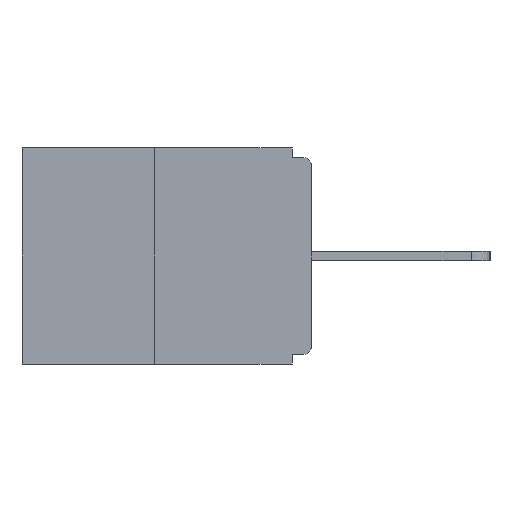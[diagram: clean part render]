
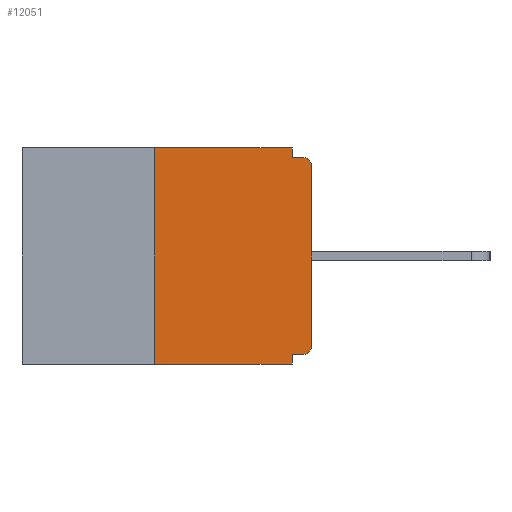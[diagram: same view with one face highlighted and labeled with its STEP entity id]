
A CAD part, left-side view. The second image highlights one B-rep face of the part: STEP entity #12051.
In plain terms, the highlighted planar face has unit normal (-1, 0, 0).
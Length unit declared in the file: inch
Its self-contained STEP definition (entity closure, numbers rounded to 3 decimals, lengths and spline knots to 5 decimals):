
#163 = ORIENTED_EDGE ( 'NONE', *, *, #1763, .F. ) ;
#190 = VERTEX_POINT ( 'NONE', #10523 ) ;
#207 = EDGE_CURVE ( 'NONE', #3106, #6853, #5096, .T. ) ;
#289 = VECTOR ( 'NONE', #5837, 39.37008 ) ;
#712 = DIRECTION ( 'NONE',  ( 0., 0., -1. ) ) ;
#765 = CARTESIAN_POINT ( 'NONE',  ( 0., 0.031, -0.015 ) ) ;
#1212 = EDGE_CURVE ( 'NONE', #190, #12961, #6072, .T. ) ;
#1265 = LINE ( 'NONE', #8754, #4879 ) ;
#1267 = ORIENTED_EDGE ( 'NONE', *, *, #207, .F. ) ;
#1307 = EDGE_CURVE ( 'NONE', #7905, #5545, #8276, .T. ) ;
#1506 = VECTOR ( 'NONE', #12488, 39.37008 ) ;
#1714 = LINE ( 'NONE', #9576, #11235 ) ;
#1763 = EDGE_CURVE ( 'NONE', #7905, #190, #1265, .T. ) ;
#2494 = DIRECTION ( 'NONE',  ( 0., 0., -1. ) ) ;
#2505 = DIRECTION ( 'NONE',  ( 0., 0., -1. ) ) ;
#2756 = CARTESIAN_POINT ( 'NONE',  ( 0., 0., -0.313 ) ) ;
#2762 = LINE ( 'NONE', #11006, #5816 ) ;
#2764 = ORIENTED_EDGE ( 'NONE', *, *, #10537, .F. ) ;
#3025 = ORIENTED_EDGE ( 'NONE', *, *, #3250, .T. ) ;
#3106 = VERTEX_POINT ( 'NONE', #765 ) ;
#3190 = LINE ( 'NONE', #3786, #289 ) ;
#3193 = VECTOR ( 'NONE', #712, 39.37008 ) ;
#3250 = EDGE_CURVE ( 'NONE', #5545, #9030, #11290, .T. ) ;
#3786 = CARTESIAN_POINT ( 'NONE',  ( 0., 0.46, -0.343 ) ) ;
#4188 = CARTESIAN_POINT ( 'NONE',  ( 0., 0.031, 0. ) ) ;
#4225 = DIRECTION ( 'NONE',  ( 0., 0., -1. ) ) ;
#4613 = EDGE_CURVE ( 'NONE', #9030, #6853, #13272, .T. ) ;
#4745 = DIRECTION ( 'NONE',  ( -1., 0., 0. ) ) ;
#4850 = CARTESIAN_POINT ( 'NONE',  ( 0., 0., 0. ) ) ;
#4879 = VECTOR ( 'NONE', #6468, 39.37008 ) ;
#4902 = ORIENTED_EDGE ( 'NONE', *, *, #4613, .T. ) ;
#4992 = CARTESIAN_POINT ( 'NONE',  ( 0., 0., -0.015 ) ) ;
#5096 = LINE ( 'NONE', #4992, #1506 ) ;
#5313 = EDGE_CURVE ( 'NONE', #11545, #3106, #13612, .T. ) ;
#5322 = EDGE_CURVE ( 'NONE', #12980, #11545, #1714, .T. ) ;
#5545 = VERTEX_POINT ( 'NONE', #2756 ) ;
#5580 = DIRECTION ( 'NONE',  ( 0., 0., 1. ) ) ;
#5816 = VECTOR ( 'NONE', #5580, 39.37008 ) ;
#5837 = DIRECTION ( 'NONE',  ( 0., -1., 0. ) ) ;
#5881 = CARTESIAN_POINT ( 'NONE',  ( 0., 0.46, 0. ) ) ;
#5884 = FACE_OUTER_BOUND ( 'NONE', #7782, .T. ) ;
#6072 = LINE ( 'NONE', #9237, #3193 ) ;
#6159 = CARTESIAN_POINT ( 'NONE',  ( 0., 0.031, -0.343 ) ) ;
#6468 = DIRECTION ( 'NONE',  ( 0., 1., 0. ) ) ;
#6846 = CARTESIAN_POINT ( 'NONE',  ( 0., 0.015, -0.03 ) ) ;
#6853 = VERTEX_POINT ( 'NONE', #8956 ) ;
#7450 = DIRECTION ( 'NONE',  ( 0., 0., -1. ) ) ;
#7782 = EDGE_LOOP ( 'NONE', ( #13099, #2764, #8736, #10281, #163, #11491, #3025, #4902, #1267, #11516 ) ) ;
#7905 = VERTEX_POINT ( 'NONE', #12425 ) ;
#8276 = CIRCLE ( 'NONE', #13742, 0.015 ) ;
#8594 = DIRECTION ( 'NONE',  ( 0., -1., 0. ) ) ;
#8736 = ORIENTED_EDGE ( 'NONE', *, *, #10135, .T. ) ;
#8754 = CARTESIAN_POINT ( 'NONE',  ( 0., 0., -0.328 ) ) ;
#8956 = CARTESIAN_POINT ( 'NONE',  ( 0., 0.015, -0.015 ) ) ;
#9006 = PLANE ( 'NONE',  #14054 ) ;
#9030 = VERTEX_POINT ( 'NONE', #11550 ) ;
#9210 = DIRECTION ( 'NONE',  ( 0., 0., 1. ) ) ;
#9237 = CARTESIAN_POINT ( 'NONE',  ( 0., 0.031, -0.343 ) ) ;
#9576 = CARTESIAN_POINT ( 'NONE',  ( 0., 0.46, 0. ) ) ;
#10135 = EDGE_CURVE ( 'NONE', #11312, #12961, #3190, .T. ) ;
#10281 = ORIENTED_EDGE ( 'NONE', *, *, #1212, .F. ) ;
#10442 = VECTOR ( 'NONE', #9210, 39.37008 ) ;
#10523 = CARTESIAN_POINT ( 'NONE',  ( 0., 0.031, -0.328 ) ) ;
#10537 = EDGE_CURVE ( 'NONE', #11312, #12980, #2762, .T. ) ;
#10743 = DIRECTION ( 'NONE',  ( -1., 0., 0. ) ) ;
#11006 = CARTESIAN_POINT ( 'NONE',  ( 0., 0.25, 0. ) ) ;
#11235 = VECTOR ( 'NONE', #8594, 39.37008 ) ;
#11290 = LINE ( 'NONE', #4850, #10442 ) ;
#11312 = VERTEX_POINT ( 'NONE', #12009 ) ;
#11491 = ORIENTED_EDGE ( 'NONE', *, *, #1307, .T. ) ;
#11516 = ORIENTED_EDGE ( 'NONE', *, *, #5313, .F. ) ;
#11545 = VERTEX_POINT ( 'NONE', #12174 ) ;
#11550 = CARTESIAN_POINT ( 'NONE',  ( 0., 0., -0.03 ) ) ;
#11565 = VECTOR ( 'NONE', #7450, 39.37008 ) ;
#11677 = CARTESIAN_POINT ( 'NONE',  ( 0., 0.25, 0. ) ) ;
#11815 = CARTESIAN_POINT ( 'NONE',  ( 0., 0.015, -0.313 ) ) ;
#11878 = AXIS2_PLACEMENT_3D ( 'NONE', #6846, #4745, #2494 ) ;
#12009 = CARTESIAN_POINT ( 'NONE',  ( 0., 0.25, -0.343 ) ) ;
#12051 = ADVANCED_FACE ( 'NONE', ( #5884 ), #9006, .F. ) ;
#12174 = CARTESIAN_POINT ( 'NONE',  ( 0., 0.031, 0. ) ) ;
#12220 = DIRECTION ( 'NONE',  ( 1., 0., 0. ) ) ;
#12425 = CARTESIAN_POINT ( 'NONE',  ( 0., 0.015, -0.328 ) ) ;
#12488 = DIRECTION ( 'NONE',  ( 0., -1., 0. ) ) ;
#12961 = VERTEX_POINT ( 'NONE', #6159 ) ;
#12980 = VERTEX_POINT ( 'NONE', #11677 ) ;
#13099 = ORIENTED_EDGE ( 'NONE', *, *, #5322, .F. ) ;
#13272 = CIRCLE ( 'NONE', #11878, 0.015 ) ;
#13612 = LINE ( 'NONE', #4188, #11565 ) ;
#13742 = AXIS2_PLACEMENT_3D ( 'NONE', #11815, #10743, #4225 ) ;
#14054 = AXIS2_PLACEMENT_3D ( 'NONE', #5881, #12220, #2505 ) ;
